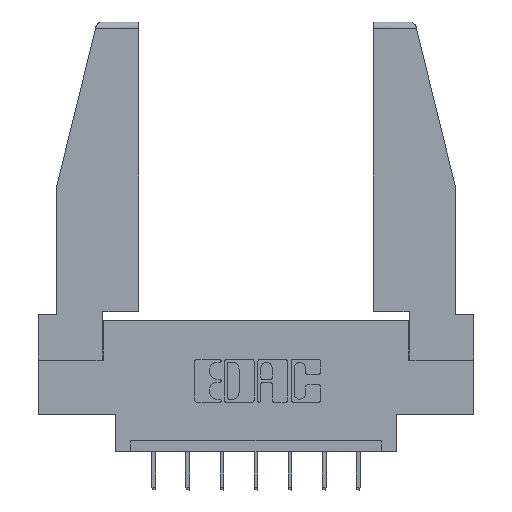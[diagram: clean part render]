
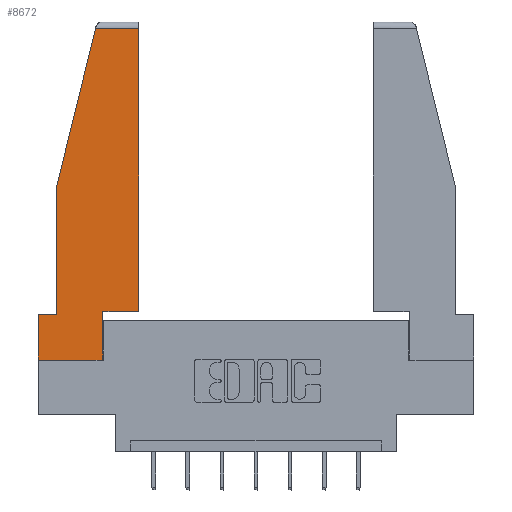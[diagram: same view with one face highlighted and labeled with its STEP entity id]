
A CAD part, top view. The second image highlights one B-rep face of the part: STEP entity #8672.
In plain terms, the highlighted planar face has unit normal (0, 0, 1).
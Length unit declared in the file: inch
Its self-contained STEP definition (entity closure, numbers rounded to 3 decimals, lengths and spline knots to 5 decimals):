
#66 = DIRECTION ( 'NONE',  ( -1., 0., 0. ) ) ;
#213 = LINE ( 'NONE', #866, #6764 ) ;
#518 = VECTOR ( 'NONE', #8690, 39.37008 ) ;
#599 = VERTEX_POINT ( 'NONE', #9939 ) ;
#732 = DIRECTION ( 'NONE',  ( 0., 1., 0. ) ) ;
#736 = DIRECTION ( 'NONE',  ( 1., 0., 0. ) ) ;
#866 = CARTESIAN_POINT ( 'NONE',  ( 0., 0.21, 0. ) ) ;
#906 = CARTESIAN_POINT ( 'NONE',  ( 0.297, 0., 0. ) ) ;
#1388 = DIRECTION ( 'NONE',  ( 0., -1., 0. ) ) ;
#1417 = VERTEX_POINT ( 'NONE', #7316 ) ;
#1809 = EDGE_CURVE ( 'NONE', #599, #8836, #8251, .T. ) ;
#2094 = ORIENTED_EDGE ( 'NONE', *, *, #12149, .T. ) ;
#2266 = EDGE_CURVE ( 'NONE', #8836, #5233, #9765, .T. ) ;
#2280 = VERTEX_POINT ( 'NONE', #3377 ) ;
#2307 = DIRECTION ( 'NONE',  ( -1., 0., 0. ) ) ;
#2850 = EDGE_CURVE ( 'NONE', #11492, #2280, #6428, .T. ) ;
#3049 = VERTEX_POINT ( 'NONE', #11232 ) ;
#3145 = CARTESIAN_POINT ( 'NONE',  ( 0.297, 0.223, 0. ) ) ;
#3203 = EDGE_CURVE ( 'NONE', #5233, #3049, #6860, .T. ) ;
#3334 = ORIENTED_EDGE ( 'NONE', *, *, #2266, .T. ) ;
#3377 = CARTESIAN_POINT ( 'NONE',  ( 0.461, 0.223, 0. ) ) ;
#4085 = LINE ( 'NONE', #9588, #518 ) ;
#4097 = LINE ( 'NONE', #11477, #11498 ) ;
#4138 = LINE ( 'NONE', #5349, #11693 ) ;
#4265 = CARTESIAN_POINT ( 'NONE',  ( 0., 1.52, 0. ) ) ;
#4296 = VECTOR ( 'NONE', #1388, 39.37008 ) ;
#5217 = CARTESIAN_POINT ( 'NONE',  ( 0.086, 0.8, 0. ) ) ;
#5233 = VERTEX_POINT ( 'NONE', #10802 ) ;
#5349 = CARTESIAN_POINT ( 'NONE',  ( 0.297, 0., 0. ) ) ;
#5387 = EDGE_CURVE ( 'NONE', #1417, #8265, #4085, .T. ) ;
#5621 = CARTESIAN_POINT ( 'NONE',  ( 0.297, 0.223, 0. ) ) ;
#6271 = FACE_OUTER_BOUND ( 'NONE', #11564, .T. ) ;
#6285 = VECTOR ( 'NONE', #2307, 39.37008 ) ;
#6428 = LINE ( 'NONE', #3145, #7324 ) ;
#6680 = AXIS2_PLACEMENT_3D ( 'NONE', #8729, #9829, #11949 ) ;
#6764 = VECTOR ( 'NONE', #66, 39.37008 ) ;
#6860 = LINE ( 'NONE', #5217, #4296 ) ;
#6973 = ORIENTED_EDGE ( 'NONE', *, *, #1809, .T. ) ;
#7091 = ORIENTED_EDGE ( 'NONE', *, *, #7351, .T. ) ;
#7316 = CARTESIAN_POINT ( 'NONE',  ( 0., 0.21, 0. ) ) ;
#7324 = VECTOR ( 'NONE', #8957, 39.37008 ) ;
#7351 = EDGE_CURVE ( 'NONE', #3049, #1417, #213, .T. ) ;
#7420 = CARTESIAN_POINT ( 'NONE',  ( 0., 0., 0. ) ) ;
#7507 = DIRECTION ( 'NONE',  ( 0., 1., 0. ) ) ;
#8059 = CARTESIAN_POINT ( 'NONE',  ( 0.2636, 1.52, 0. ) ) ;
#8188 = DIRECTION ( 'NONE',  ( -0.239, -0.971, 0. ) ) ;
#8251 = LINE ( 'NONE', #4265, #6285 ) ;
#8265 = VERTEX_POINT ( 'NONE', #7420 ) ;
#8523 = ORIENTED_EDGE ( 'NONE', *, *, #12234, .T. ) ;
#8582 = ORIENTED_EDGE ( 'NONE', *, *, #2850, .T. ) ;
#8672 = ADVANCED_FACE ( 'NONE', ( #6271 ), #11696, .T. ) ;
#8690 = DIRECTION ( 'NONE',  ( 0., -1., 0. ) ) ;
#8729 = CARTESIAN_POINT ( 'NONE',  ( 0., 0., 0. ) ) ;
#8836 = VERTEX_POINT ( 'NONE', #8059 ) ;
#8957 = DIRECTION ( 'NONE',  ( 1., 0., 0. ) ) ;
#9588 = CARTESIAN_POINT ( 'NONE',  ( 0., 0.21, 0. ) ) ;
#9765 = LINE ( 'NONE', #11172, #12175 ) ;
#9829 = DIRECTION ( 'NONE',  ( 0., 0., 1. ) ) ;
#9939 = CARTESIAN_POINT ( 'NONE',  ( 0.461, 1.52, 0. ) ) ;
#10285 = EDGE_CURVE ( 'NONE', #11381, #11492, #4138, .T. ) ;
#10415 = ORIENTED_EDGE ( 'NONE', *, *, #3203, .T. ) ;
#10617 = VECTOR ( 'NONE', #736, 39.37008 ) ;
#10802 = CARTESIAN_POINT ( 'NONE',  ( 0.086, 0.8, 0. ) ) ;
#11107 = CARTESIAN_POINT ( 'NONE',  ( 0., 0., 0. ) ) ;
#11172 = CARTESIAN_POINT ( 'NONE',  ( 0.271, 1.55, 0. ) ) ;
#11207 = LINE ( 'NONE', #11107, #10617 ) ;
#11232 = CARTESIAN_POINT ( 'NONE',  ( 0.086, 0.21, 0. ) ) ;
#11381 = VERTEX_POINT ( 'NONE', #906 ) ;
#11477 = CARTESIAN_POINT ( 'NONE',  ( 0.461, 0.223, 0. ) ) ;
#11492 = VERTEX_POINT ( 'NONE', #5621 ) ;
#11498 = VECTOR ( 'NONE', #7507, 39.37008 ) ;
#11564 = EDGE_LOOP ( 'NONE', ( #8523, #6973, #3334, #10415, #7091, #12337, #2094, #12061, #8582 ) ) ;
#11693 = VECTOR ( 'NONE', #732, 39.37008 ) ;
#11696 = PLANE ( 'NONE',  #6680 ) ;
#11949 = DIRECTION ( 'NONE',  ( 1., 0., 0. ) ) ;
#12061 = ORIENTED_EDGE ( 'NONE', *, *, #10285, .T. ) ;
#12149 = EDGE_CURVE ( 'NONE', #8265, #11381, #11207, .T. ) ;
#12175 = VECTOR ( 'NONE', #8188, 39.37008 ) ;
#12234 = EDGE_CURVE ( 'NONE', #2280, #599, #4097, .T. ) ;
#12337 = ORIENTED_EDGE ( 'NONE', *, *, #5387, .T. ) ;
